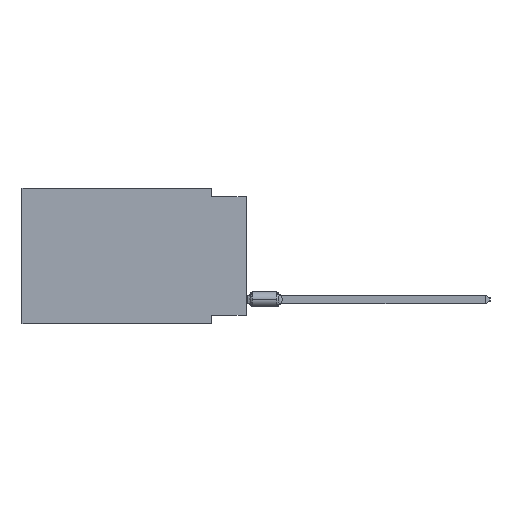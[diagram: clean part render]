
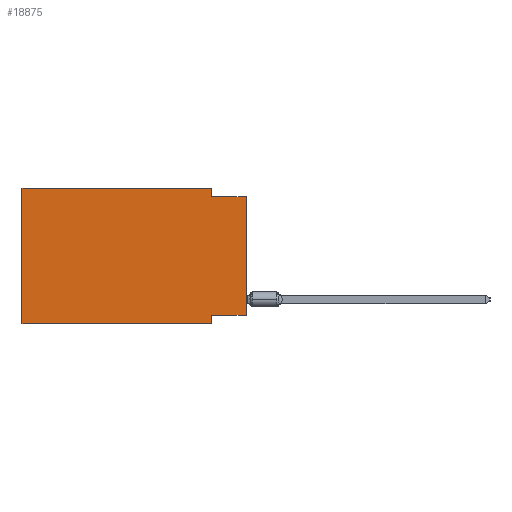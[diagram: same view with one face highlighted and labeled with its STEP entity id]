
A CAD part, left-side view. The second image highlights one B-rep face of the part: STEP entity #18875.
In plain terms, the highlighted planar face has unit normal (-1, 0, 0).
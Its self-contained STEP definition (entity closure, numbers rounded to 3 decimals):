
#2458 = CARTESIAN_POINT ( 'NONE',  ( 0., 16.383, 0. ) ) ;
#3298 = ORIENTED_EDGE ( 'NONE', *, *, #20217, .F. ) ;
#4544 = VECTOR ( 'NONE', #75904, 1000. ) ;
#5824 = CARTESIAN_POINT ( 'NONE',  ( 0., 0., -9.271 ) ) ;
#6048 = ORIENTED_EDGE ( 'NONE', *, *, #7619, .T. ) ;
#6984 = LINE ( 'NONE', #5824, #37722 ) ;
#7176 = CARTESIAN_POINT ( 'NONE',  ( 0., 2.54, -9.271 ) ) ;
#7619 = EDGE_CURVE ( 'NONE', #46487, #72163, #10144, .T. ) ;
#7650 = EDGE_CURVE ( 'NONE', #41131, #72163, #16080, .T. ) ;
#9345 = DIRECTION ( 'NONE',  ( 0., 0., 1. ) ) ;
#9746 = CARTESIAN_POINT ( 'NONE',  ( 0., 0., 0. ) ) ;
#10144 = LINE ( 'NONE', #9746, #40641 ) ;
#11451 = VECTOR ( 'NONE', #40316, 1000. ) ;
#14849 = ORIENTED_EDGE ( 'NONE', *, *, #38490, .F. ) ;
#16080 = LINE ( 'NONE', #27584, #11451 ) ;
#17633 = LINE ( 'NONE', #72043, #60949 ) ;
#18047 = ORIENTED_EDGE ( 'NONE', *, *, #59571, .F. ) ;
#18119 = CARTESIAN_POINT ( 'NONE',  ( 0., 16.383, 0. ) ) ;
#18130 = DIRECTION ( 'NONE',  ( 0., 1., 0. ) ) ;
#18509 = DIRECTION ( 'NONE',  ( 1., 0., 0. ) ) ;
#18875 = ADVANCED_FACE ( 'NONE', ( #41554 ), #65782, .F. ) ;
#20217 = EDGE_CURVE ( 'NONE', #46487, #56738, #6984, .T. ) ;
#22643 = ORIENTED_EDGE ( 'NONE', *, *, #26469, .F. ) ;
#23055 = CARTESIAN_POINT ( 'NONE',  ( 0., 2.54, -9.906 ) ) ;
#23449 = CARTESIAN_POINT ( 'NONE',  ( 0., 0., -0.635 ) ) ;
#25293 = CARTESIAN_POINT ( 'NONE',  ( 0., 2.54, -9.906 ) ) ;
#25900 = LINE ( 'NONE', #31859, #29201 ) ;
#26469 = EDGE_CURVE ( 'NONE', #42800, #46413, #56848, .T. ) ;
#27584 = CARTESIAN_POINT ( 'NONE',  ( 0., 0., -0.635 ) ) ;
#29201 = VECTOR ( 'NONE', #30299, 1000. ) ;
#29455 = CARTESIAN_POINT ( 'NONE',  ( 0., 16.383, -9.906 ) ) ;
#30299 = DIRECTION ( 'NONE',  ( 0., -1., 0. ) ) ;
#31859 = CARTESIAN_POINT ( 'NONE',  ( 0., 16.383, -9.906 ) ) ;
#37722 = VECTOR ( 'NONE', #18130, 1000. ) ;
#38326 = DIRECTION ( 'NONE',  ( 0., 0., -1. ) ) ;
#38490 = EDGE_CURVE ( 'NONE', #56738, #72653, #78251, .T. ) ;
#39600 = VECTOR ( 'NONE', #38326, 1000. ) ;
#40316 = DIRECTION ( 'NONE',  ( 0., -1., 0. ) ) ;
#40641 = VECTOR ( 'NONE', #9345, 1000. ) ;
#41131 = VERTEX_POINT ( 'NONE', #42634 ) ;
#41554 = FACE_OUTER_BOUND ( 'NONE', #45344, .T. ) ;
#41850 = DIRECTION ( 'NONE',  ( 0., -1., 0. ) ) ;
#42265 = CARTESIAN_POINT ( 'NONE',  ( 0., 2.54, 0. ) ) ;
#42634 = CARTESIAN_POINT ( 'NONE',  ( 0., 2.54, -0.635 ) ) ;
#42800 = VERTEX_POINT ( 'NONE', #29455 ) ;
#45344 = EDGE_LOOP ( 'NONE', ( #6048, #52441, #55175, #18047, #22643, #68953, #14849, #3298 ) ) ;
#46413 = VERTEX_POINT ( 'NONE', #69481 ) ;
#46487 = VERTEX_POINT ( 'NONE', #77018 ) ;
#46490 = VECTOR ( 'NONE', #48444, 1000. ) ;
#48444 = DIRECTION ( 'NONE',  ( 0., 0., -1. ) ) ;
#50627 = CARTESIAN_POINT ( 'NONE',  ( 0., 2.54, 0. ) ) ;
#52441 = ORIENTED_EDGE ( 'NONE', *, *, #7650, .F. ) ;
#54220 = VERTEX_POINT ( 'NONE', #42265 ) ;
#55175 = ORIENTED_EDGE ( 'NONE', *, *, #60485, .F. ) ;
#56738 = VERTEX_POINT ( 'NONE', #7176 ) ;
#56848 = LINE ( 'NONE', #2458, #4544 ) ;
#59571 = EDGE_CURVE ( 'NONE', #46413, #54220, #17633, .T. ) ;
#59606 = EDGE_CURVE ( 'NONE', #42800, #72653, #25900, .T. ) ;
#60485 = EDGE_CURVE ( 'NONE', #54220, #41131, #74089, .T. ) ;
#60949 = VECTOR ( 'NONE', #41850, 1000. ) ;
#65393 = DIRECTION ( 'NONE',  ( 0., 0., -1. ) ) ;
#65782 = PLANE ( 'NONE',  #71875 ) ;
#68953 = ORIENTED_EDGE ( 'NONE', *, *, #59606, .T. ) ;
#69481 = CARTESIAN_POINT ( 'NONE',  ( 0., 16.383, 0. ) ) ;
#71875 = AXIS2_PLACEMENT_3D ( 'NONE', #18119, #18509, #65393 ) ;
#72043 = CARTESIAN_POINT ( 'NONE',  ( 0., 16.383, 0. ) ) ;
#72163 = VERTEX_POINT ( 'NONE', #23449 ) ;
#72653 = VERTEX_POINT ( 'NONE', #25293 ) ;
#74089 = LINE ( 'NONE', #50627, #39600 ) ;
#75904 = DIRECTION ( 'NONE',  ( 0., 0., 1. ) ) ;
#77018 = CARTESIAN_POINT ( 'NONE',  ( 0., 0., -9.271 ) ) ;
#78251 = LINE ( 'NONE', #23055, #46490 ) ;
